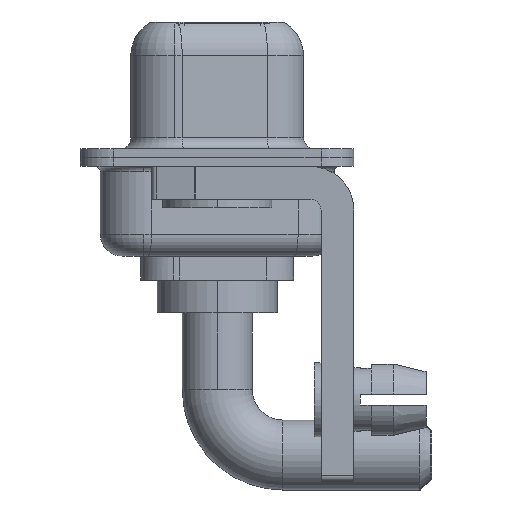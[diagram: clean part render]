
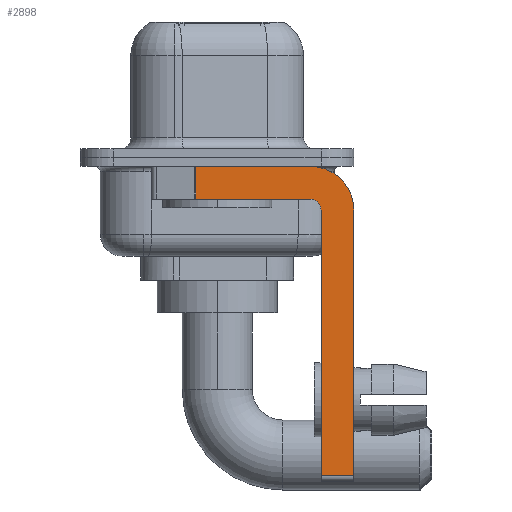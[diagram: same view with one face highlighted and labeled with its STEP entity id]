
A CAD part, left-side view. The second image highlights one B-rep face of the part: STEP entity #2898.
In plain terms, the highlighted planar face has unit normal (-1, 0, 0).
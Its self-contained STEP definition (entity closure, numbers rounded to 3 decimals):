
#482 = VECTOR ( 'NONE', #16163, 1000. ) ;
#528 = AXIS2_PLACEMENT_3D ( 'NONE', #3319, #10695, #6842 ) ;
#830 = VECTOR ( 'NONE', #13349, 1000. ) ;
#1120 = LINE ( 'NONE', #9878, #482 ) ;
#1315 = PLANE ( 'NONE',  #9153 ) ;
#1374 = CARTESIAN_POINT ( 'NONE',  ( -2.9, -4.75, -14.55 ) ) ;
#1579 = CARTESIAN_POINT ( 'NONE',  ( -2.9, 0.978, -0.4 ) ) ;
#1617 = FACE_OUTER_BOUND ( 'NONE', #14158, .T. ) ;
#1663 = CARTESIAN_POINT ( 'NONE',  ( -2.9, -6.25, -2.4 ) ) ;
#1704 = DIRECTION ( 'NONE',  ( 0., -1., 0. ) ) ;
#1858 = LINE ( 'NONE', #10467, #2703 ) ;
#2201 = VECTOR ( 'NONE', #14923, 1000. ) ;
#2564 = ORIENTED_EDGE ( 'NONE', *, *, #4596, .T. ) ;
#2703 = VECTOR ( 'NONE', #1704, 1000. ) ;
#2898 = ADVANCED_FACE ( 'NONE', ( #1617 ), #1315, .F. ) ;
#3020 = EDGE_CURVE ( 'NONE', #7484, #5775, #6530, .T. ) ;
#3319 = CARTESIAN_POINT ( 'NONE',  ( -2.9, -4.25, -2.4 ) ) ;
#3368 = CARTESIAN_POINT ( 'NONE',  ( -2.9, -4.25, -1.9 ) ) ;
#3375 = DIRECTION ( 'NONE',  ( -1., 0., 0. ) ) ;
#4029 = CARTESIAN_POINT ( 'NONE',  ( -2.9, -4.75, -2.4 ) ) ;
#4388 = ORIENTED_EDGE ( 'NONE', *, *, #10451, .F. ) ;
#4519 = CARTESIAN_POINT ( 'NONE',  ( -2.9, -4.25, -14.55 ) ) ;
#4596 = EDGE_CURVE ( 'NONE', #5327, #12728, #14410, .T. ) ;
#5327 = VERTEX_POINT ( 'NONE', #1374 ) ;
#5632 = CARTESIAN_POINT ( 'NONE',  ( -2.9, -6.25, -2.4 ) ) ;
#5775 = VERTEX_POINT ( 'NONE', #1663 ) ;
#5816 = VERTEX_POINT ( 'NONE', #1579 ) ;
#5991 = DIRECTION ( 'NONE',  ( 0., 1., 0. ) ) ;
#6304 = CARTESIAN_POINT ( 'NONE',  ( -2.9, -4.25, -2.4 ) ) ;
#6379 = VECTOR ( 'NONE', #15605, 1000. ) ;
#6530 = CIRCLE ( 'NONE', #528, 2. ) ;
#6842 = DIRECTION ( 'NONE',  ( 0., 0., -1. ) ) ;
#6974 = EDGE_CURVE ( 'NONE', #5327, #7800, #1120, .T. ) ;
#7063 = CARTESIAN_POINT ( 'NONE',  ( -2.9, -4.25, -2.4 ) ) ;
#7319 = VECTOR ( 'NONE', #5991, 1000. ) ;
#7484 = VERTEX_POINT ( 'NONE', #14664 ) ;
#7784 = ORIENTED_EDGE ( 'NONE', *, *, #3020, .F. ) ;
#7800 = VERTEX_POINT ( 'NONE', #4029 ) ;
#8427 = CIRCLE ( 'NONE', #12623, 0.5 ) ;
#9153 = AXIS2_PLACEMENT_3D ( 'NONE', #6304, #11302, #15056 ) ;
#9383 = VERTEX_POINT ( 'NONE', #11065 ) ;
#9878 = CARTESIAN_POINT ( 'NONE',  ( -2.9, -4.75, -14.8 ) ) ;
#10451 = EDGE_CURVE ( 'NONE', #15652, #9383, #15882, .T. ) ;
#10467 = CARTESIAN_POINT ( 'NONE',  ( -2.9, 3., -0.4 ) ) ;
#10695 = DIRECTION ( 'NONE',  ( 1., 0., 0. ) ) ;
#10911 = DIRECTION ( 'NONE',  ( 0., 0., 1. ) ) ;
#11065 = CARTESIAN_POINT ( 'NONE',  ( -2.9, 0.978, -1.9 ) ) ;
#11088 = LINE ( 'NONE', #11251, #2201 ) ;
#11251 = CARTESIAN_POINT ( 'NONE',  ( -2.9, 0.978, -1.9 ) ) ;
#11302 = DIRECTION ( 'NONE',  ( 1., 0., 0. ) ) ;
#11394 = ORIENTED_EDGE ( 'NONE', *, *, #12777, .F. ) ;
#11856 = LINE ( 'NONE', #5632, #6379 ) ;
#12495 = CARTESIAN_POINT ( 'NONE',  ( -2.9, -4.25, -1.9 ) ) ;
#12623 = AXIS2_PLACEMENT_3D ( 'NONE', #7063, #3375, #10911 ) ;
#12639 = ORIENTED_EDGE ( 'NONE', *, *, #15298, .F. ) ;
#12728 = VERTEX_POINT ( 'NONE', #14578 ) ;
#12777 = EDGE_CURVE ( 'NONE', #7800, #15652, #8427, .T. ) ;
#13349 = DIRECTION ( 'NONE',  ( 0., -1., 0. ) ) ;
#13372 = ORIENTED_EDGE ( 'NONE', *, *, #15356, .F. ) ;
#14158 = EDGE_LOOP ( 'NONE', ( #12639, #14372, #4388, #11394, #14601, #2564, #13372, #7784 ) ) ;
#14372 = ORIENTED_EDGE ( 'NONE', *, *, #16088, .T. ) ;
#14410 = LINE ( 'NONE', #4519, #830 ) ;
#14578 = CARTESIAN_POINT ( 'NONE',  ( -2.9, -6.25, -14.55 ) ) ;
#14601 = ORIENTED_EDGE ( 'NONE', *, *, #6974, .F. ) ;
#14664 = CARTESIAN_POINT ( 'NONE',  ( -2.9, -4.25, -0.4 ) ) ;
#14923 = DIRECTION ( 'NONE',  ( 0., 0., -1. ) ) ;
#15056 = DIRECTION ( 'NONE',  ( 0., 0., -1. ) ) ;
#15298 = EDGE_CURVE ( 'NONE', #5816, #7484, #1858, .T. ) ;
#15356 = EDGE_CURVE ( 'NONE', #5775, #12728, #11856, .T. ) ;
#15605 = DIRECTION ( 'NONE',  ( 0., 0., -1. ) ) ;
#15652 = VERTEX_POINT ( 'NONE', #12495 ) ;
#15882 = LINE ( 'NONE', #3368, #7319 ) ;
#16088 = EDGE_CURVE ( 'NONE', #5816, #9383, #11088, .T. ) ;
#16163 = DIRECTION ( 'NONE',  ( 0., 0., 1. ) ) ;
